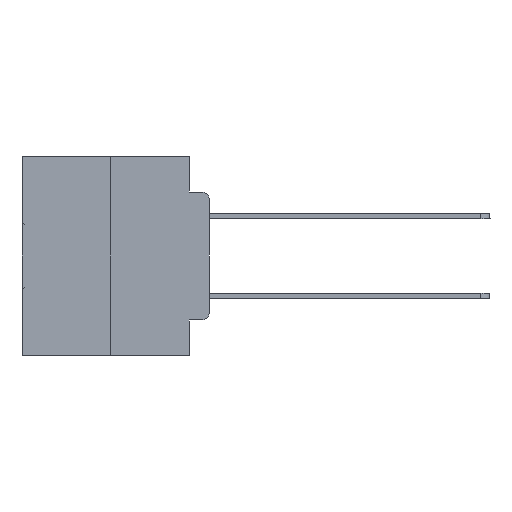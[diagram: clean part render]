
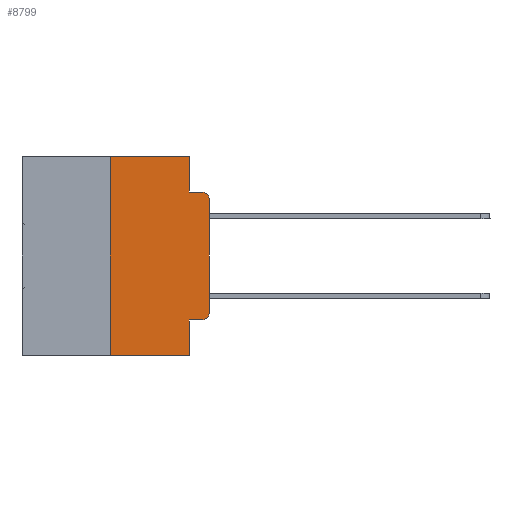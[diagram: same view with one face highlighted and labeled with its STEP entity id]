
A CAD part, left-side view. The second image highlights one B-rep face of the part: STEP entity #8799.
In plain terms, the highlighted planar face has unit normal (-1, 0, 0).
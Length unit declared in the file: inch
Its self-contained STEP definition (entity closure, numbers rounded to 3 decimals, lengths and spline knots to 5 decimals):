
#79 = CARTESIAN_POINT ( 'NONE',  ( 0., 0.02, -0.3915 ) ) ;
#317 = EDGE_CURVE ( 'NONE', #12900, #11009, #21360, .T. ) ;
#398 = DIRECTION ( 'NONE',  ( -1., 0., 0. ) ) ;
#597 = ORIENTED_EDGE ( 'NONE', *, *, #7160, .T. ) ;
#1193 = VERTEX_POINT ( 'NONE', #11945 ) ;
#1997 = DIRECTION ( 'NONE',  ( 0., -1., 0. ) ) ;
#2326 = ORIENTED_EDGE ( 'NONE', *, *, #20658, .T. ) ;
#2502 = LINE ( 'NONE', #30355, #7839 ) ;
#2874 = DIRECTION ( 'NONE',  ( 0., 0., -1. ) ) ;
#2992 = FACE_OUTER_BOUND ( 'NONE', #20978, .T. ) ;
#3147 = AXIS2_PLACEMENT_3D ( 'NONE', #16035, #21501, #31085 ) ;
#3903 = CARTESIAN_POINT ( 'NONE',  ( 0., 0.051, -0.4115 ) ) ;
#4200 = CARTESIAN_POINT ( 'NONE',  ( 0., 0.25, 0. ) ) ;
#4584 = VERTEX_POINT ( 'NONE', #19015 ) ;
#5162 = DIRECTION ( 'NONE',  ( 0., -1., 0. ) ) ;
#5604 = VERTEX_POINT ( 'NONE', #29519 ) ;
#6699 = CARTESIAN_POINT ( 'NONE',  ( 0., 0.25, -0.5 ) ) ;
#6832 = DIRECTION ( 'NONE',  ( 0., -1., 0. ) ) ;
#6986 = CARTESIAN_POINT ( 'NONE',  ( 0., 0.473, 0. ) ) ;
#7160 = EDGE_CURVE ( 'NONE', #12900, #24112, #26743, .T. ) ;
#7560 = VERTEX_POINT ( 'NONE', #17370 ) ;
#7839 = VECTOR ( 'NONE', #5162, 39.37008 ) ;
#7877 = EDGE_CURVE ( 'NONE', #4584, #24963, #30154, .T. ) ;
#8146 = CARTESIAN_POINT ( 'NONE',  ( 0., 0.473, 0. ) ) ;
#8799 = ADVANCED_FACE ( 'NONE', ( #2992 ), #20773, .F. ) ;
#9141 = CARTESIAN_POINT ( 'NONE',  ( 0., 0.02, -0.0885 ) ) ;
#9366 = CARTESIAN_POINT ( 'NONE',  ( 0., 0.02, -0.4115 ) ) ;
#9823 = ORIENTED_EDGE ( 'NONE', *, *, #16158, .T. ) ;
#11009 = VERTEX_POINT ( 'NONE', #18061 ) ;
#11221 = CARTESIAN_POINT ( 'NONE',  ( 0., 0.051, 0. ) ) ;
#11284 = VECTOR ( 'NONE', #1997, 39.37008 ) ;
#11383 = ORIENTED_EDGE ( 'NONE', *, *, #22058, .F. ) ;
#11392 = CARTESIAN_POINT ( 'NONE',  ( 0., 0.051, 0. ) ) ;
#11760 = VERTEX_POINT ( 'NONE', #6699 ) ;
#11945 = CARTESIAN_POINT ( 'NONE',  ( 0., 0.25, 0. ) ) ;
#11965 = CARTESIAN_POINT ( 'NONE',  ( 0., 0.051, -0.4115 ) ) ;
#12465 = ORIENTED_EDGE ( 'NONE', *, *, #29556, .F. ) ;
#12467 = ORIENTED_EDGE ( 'NONE', *, *, #317, .F. ) ;
#12900 = VERTEX_POINT ( 'NONE', #3903 ) ;
#14153 = LINE ( 'NONE', #4200, #30379 ) ;
#14460 = VERTEX_POINT ( 'NONE', #32266 ) ;
#14953 = VECTOR ( 'NONE', #30666, 39.37008 ) ;
#15624 = ORIENTED_EDGE ( 'NONE', *, *, #7877, .T. ) ;
#15780 = DIRECTION ( 'NONE',  ( 0., 0., -1. ) ) ;
#16035 = CARTESIAN_POINT ( 'NONE',  ( 0., 0.02, -0.1085 ) ) ;
#16158 = EDGE_CURVE ( 'NONE', #11760, #11009, #2502, .T. ) ;
#16662 = DIRECTION ( 'NONE',  ( 0., 0., 1. ) ) ;
#17047 = ORIENTED_EDGE ( 'NONE', *, *, #18951, .F. ) ;
#17370 = CARTESIAN_POINT ( 'NONE',  ( 0., 0.051, 0. ) ) ;
#17733 = VECTOR ( 'NONE', #19020, 39.37008 ) ;
#17865 = EDGE_CURVE ( 'NONE', #24112, #5604, #31192, .T. ) ;
#18061 = CARTESIAN_POINT ( 'NONE',  ( 0., 0.051, -0.5 ) ) ;
#18681 = LINE ( 'NONE', #11221, #32329 ) ;
#18951 = EDGE_CURVE ( 'NONE', #7560, #14460, #18681, .T. ) ;
#19015 = CARTESIAN_POINT ( 'NONE',  ( 0., 0., -0.1085 ) ) ;
#19020 = DIRECTION ( 'NONE',  ( 0., 0., -1. ) ) ;
#20026 = DIRECTION ( 'NONE',  ( 0., 0., 1. ) ) ;
#20069 = VECTOR ( 'NONE', #6832, 39.37008 ) ;
#20097 = AXIS2_PLACEMENT_3D ( 'NONE', #79, #398, #2874 ) ;
#20658 = EDGE_CURVE ( 'NONE', #5604, #4584, #30281, .T. ) ;
#20773 = PLANE ( 'NONE',  #22274 ) ;
#20978 = EDGE_LOOP ( 'NONE', ( #2326, #15624, #11383, #17047, #12465, #29917, #9823, #12467, #597, #31914 ) ) ;
#21313 = VECTOR ( 'NONE', #20026, 39.37008 ) ;
#21351 = DIRECTION ( 'NONE',  ( 0., 0., -1. ) ) ;
#21360 = LINE ( 'NONE', #11392, #17733 ) ;
#21501 = DIRECTION ( 'NONE',  ( -1., 0., 0. ) ) ;
#22058 = EDGE_CURVE ( 'NONE', #14460, #24963, #30339, .T. ) ;
#22274 = AXIS2_PLACEMENT_3D ( 'NONE', #8146, #28376, #15780 ) ;
#24112 = VERTEX_POINT ( 'NONE', #9366 ) ;
#24963 = VERTEX_POINT ( 'NONE', #9141 ) ;
#26042 = CARTESIAN_POINT ( 'NONE',  ( 0., 0.051, -0.0885 ) ) ;
#26743 = LINE ( 'NONE', #11965, #20069 ) ;
#27220 = LINE ( 'NONE', #6986, #11284 ) ;
#27322 = CARTESIAN_POINT ( 'NONE',  ( 0., 0., 0. ) ) ;
#28376 = DIRECTION ( 'NONE',  ( 1., 0., 0. ) ) ;
#29519 = CARTESIAN_POINT ( 'NONE',  ( 0., 0., -0.3915 ) ) ;
#29556 = EDGE_CURVE ( 'NONE', #1193, #7560, #27220, .T. ) ;
#29917 = ORIENTED_EDGE ( 'NONE', *, *, #30196, .F. ) ;
#30154 = CIRCLE ( 'NONE', #3147, 0.02 ) ;
#30196 = EDGE_CURVE ( 'NONE', #11760, #1193, #14153, .T. ) ;
#30281 = LINE ( 'NONE', #27322, #21313 ) ;
#30339 = LINE ( 'NONE', #26042, #14953 ) ;
#30355 = CARTESIAN_POINT ( 'NONE',  ( 0., 0.473, -0.5 ) ) ;
#30379 = VECTOR ( 'NONE', #16662, 39.37008 ) ;
#30666 = DIRECTION ( 'NONE',  ( 0., -1., 0. ) ) ;
#31085 = DIRECTION ( 'NONE',  ( 0., 0., -1. ) ) ;
#31192 = CIRCLE ( 'NONE', #20097, 0.02 ) ;
#31914 = ORIENTED_EDGE ( 'NONE', *, *, #17865, .T. ) ;
#32266 = CARTESIAN_POINT ( 'NONE',  ( 0., 0.051, -0.0885 ) ) ;
#32329 = VECTOR ( 'NONE', #21351, 39.37008 ) ;
